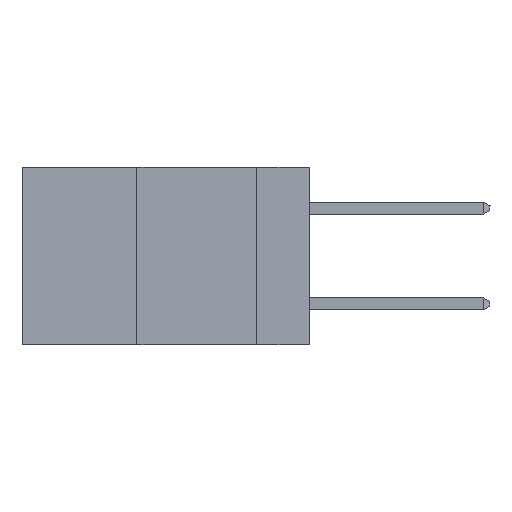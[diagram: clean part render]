
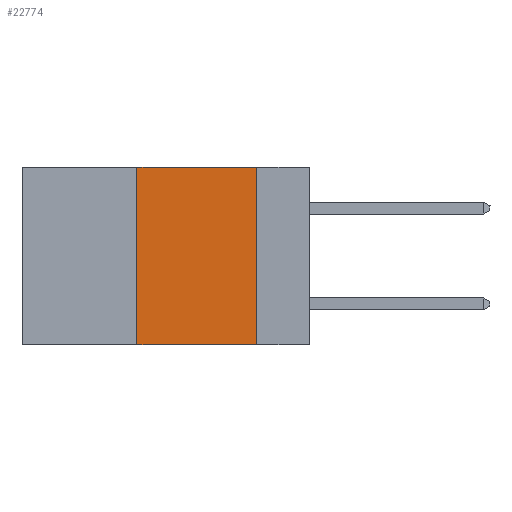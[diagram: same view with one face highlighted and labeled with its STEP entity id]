
A CAD part, left-side view. The second image highlights one B-rep face of the part: STEP entity #22774.
In plain terms, the highlighted planar face has unit normal (-1, 0, 0).
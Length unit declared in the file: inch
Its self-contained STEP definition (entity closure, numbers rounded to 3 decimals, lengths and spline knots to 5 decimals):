
#703 = EDGE_CURVE ( 'NONE', #34204, #13589, #35425, .T. ) ;
#2708 = DIRECTION ( 'NONE',  ( 0., 0., 1. ) ) ;
#3993 = LINE ( 'NONE', #13116, #29405 ) ;
#4749 = FACE_OUTER_BOUND ( 'NONE', #21606, .T. ) ;
#6032 = LINE ( 'NONE', #41531, #28318 ) ;
#12644 = CARTESIAN_POINT ( 'NONE',  ( 0., 0.6, -0.37 ) ) ;
#13116 = CARTESIAN_POINT ( 'NONE',  ( 0., 0.36, 0. ) ) ;
#13589 = VERTEX_POINT ( 'NONE', #39863 ) ;
#19203 = ORIENTED_EDGE ( 'NONE', *, *, #703, .F. ) ;
#19239 = VERTEX_POINT ( 'NONE', #38471 ) ;
#19301 = DIRECTION ( 'NONE',  ( 0., 0., -1. ) ) ;
#19458 = EDGE_CURVE ( 'NONE', #19239, #34204, #6032, .T. ) ;
#20074 = ORIENTED_EDGE ( 'NONE', *, *, #19458, .F. ) ;
#20415 = DIRECTION ( 'NONE',  ( 1., 0., 0. ) ) ;
#21606 = EDGE_LOOP ( 'NONE', ( #19203, #20074, #31523, #24734 ) ) ;
#22032 = DIRECTION ( 'NONE',  ( 0., -1., 0. ) ) ;
#22774 = ADVANCED_FACE ( 'NONE', ( #4749 ), #27260, .F. ) ;
#24028 = VECTOR ( 'NONE', #19301, 39.37008 ) ;
#24734 = ORIENTED_EDGE ( 'NONE', *, *, #42681, .T. ) ;
#25105 = VECTOR ( 'NONE', #26251, 39.37008 ) ;
#26251 = DIRECTION ( 'NONE',  ( 0., -1., 0. ) ) ;
#26458 = CARTESIAN_POINT ( 'NONE',  ( 0., 0.11, 0. ) ) ;
#27121 = DIRECTION ( 'NONE',  ( 0., 0., -1. ) ) ;
#27260 = PLANE ( 'NONE',  #33470 ) ;
#28318 = VECTOR ( 'NONE', #22032, 39.37008 ) ;
#28517 = CARTESIAN_POINT ( 'NONE',  ( 0., 0.36, -0.37 ) ) ;
#29405 = VECTOR ( 'NONE', #2708, 39.37008 ) ;
#31523 = ORIENTED_EDGE ( 'NONE', *, *, #36574, .F. ) ;
#31561 = VERTEX_POINT ( 'NONE', #28517 ) ;
#33182 = CARTESIAN_POINT ( 'NONE',  ( 0., 0.6, 0. ) ) ;
#33470 = AXIS2_PLACEMENT_3D ( 'NONE', #33182, #20415, #27121 ) ;
#34204 = VERTEX_POINT ( 'NONE', #26458 ) ;
#35425 = LINE ( 'NONE', #42345, #24028 ) ;
#36574 = EDGE_CURVE ( 'NONE', #31561, #19239, #3993, .T. ) ;
#38471 = CARTESIAN_POINT ( 'NONE',  ( 0., 0.36, 0. ) ) ;
#39863 = CARTESIAN_POINT ( 'NONE',  ( 0., 0.11, -0.37 ) ) ;
#40048 = LINE ( 'NONE', #12644, #25105 ) ;
#41531 = CARTESIAN_POINT ( 'NONE',  ( 0., 0.6, 0. ) ) ;
#42345 = CARTESIAN_POINT ( 'NONE',  ( 0., 0.11, 0. ) ) ;
#42681 = EDGE_CURVE ( 'NONE', #31561, #13589, #40048, .T. ) ;
